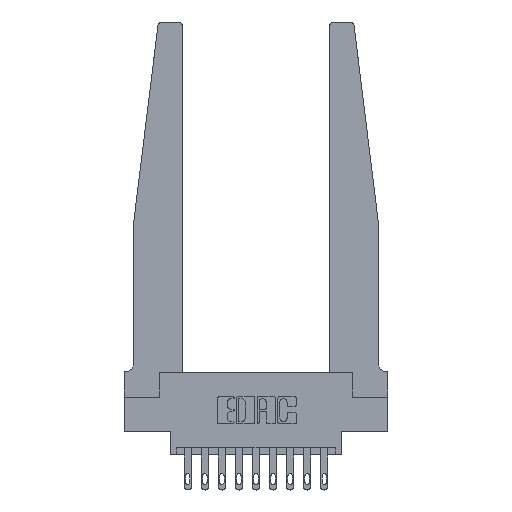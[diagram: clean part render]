
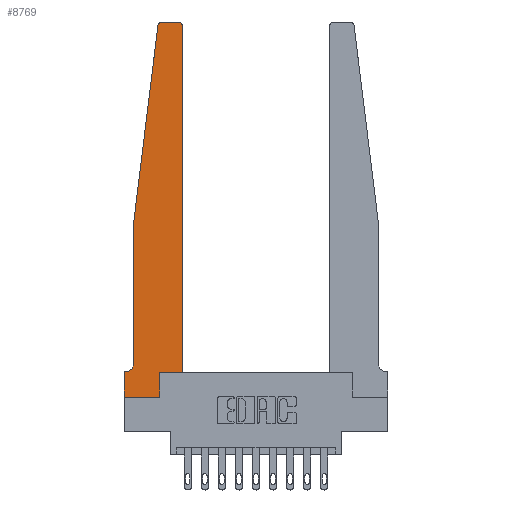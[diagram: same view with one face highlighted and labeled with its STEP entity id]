
A CAD part, top view. The second image highlights one B-rep face of the part: STEP entity #8769.
In plain terms, the highlighted planar face has unit normal (0, 0, 1).
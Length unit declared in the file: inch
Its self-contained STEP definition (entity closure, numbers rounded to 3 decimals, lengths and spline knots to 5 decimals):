
#278 = CARTESIAN_POINT ( 'NONE',  ( 0., 0.1875, 0.37 ) ) ;
#297 = CARTESIAN_POINT ( 'NONE',  ( 0.24675, 2.72367, 0.37 ) ) ;
#384 = DIRECTION ( 'NONE',  ( 0., 1., 0. ) ) ;
#623 = VERTEX_POINT ( 'NONE', #12539 ) ;
#627 = CARTESIAN_POINT ( 'NONE',  ( 0.425, 2.72, 0.37 ) ) ;
#632 = EDGE_CURVE ( 'NONE', #8275, #15040, #13407, .T. ) ;
#666 = VECTOR ( 'NONE', #12272, 39.37008 ) ;
#697 = CARTESIAN_POINT ( 'NONE',  ( 0.2605, 0.18, 0.37 ) ) ;
#800 = VERTEX_POINT ( 'NONE', #627 ) ;
#1110 = CIRCLE ( 'NONE', #4379, 0.05 ) ;
#1800 = DIRECTION ( 'NONE',  ( 0., 0., 1. ) ) ;
#1875 = CARTESIAN_POINT ( 'NONE',  ( 0.015, 0.1875, 0.37 ) ) ;
#2481 = CIRCLE ( 'NONE', #14041, 0.03 ) ;
#2810 = CARTESIAN_POINT ( 'NONE',  ( 0.395, 2.75, 0.37 ) ) ;
#2941 = ORIENTED_EDGE ( 'NONE', *, *, #6057, .T. ) ;
#2956 = DIRECTION ( 'NONE',  ( 1., 0., 0. ) ) ;
#3009 = CARTESIAN_POINT ( 'NONE',  ( 0.395, 2.72, 0.37 ) ) ;
#3151 = VECTOR ( 'NONE', #12362, 39.37008 ) ;
#3582 = CARTESIAN_POINT ( 'NONE',  ( 0.2605, 0.18, 0.37 ) ) ;
#3912 = AXIS2_PLACEMENT_3D ( 'NONE', #4189, #11306, #2956 ) ;
#4028 = ORIENTED_EDGE ( 'NONE', *, *, #6815, .T. ) ;
#4189 = CARTESIAN_POINT ( 'NONE',  ( 0., 0.1875, 0.37 ) ) ;
#4379 = AXIS2_PLACEMENT_3D ( 'NONE', #13967, #10591, #9338 ) ;
#4678 = LINE ( 'NONE', #3582, #14267 ) ;
#4982 = ORIENTED_EDGE ( 'NONE', *, *, #15145, .T. ) ;
#5058 = EDGE_CURVE ( 'NONE', #623, #11963, #1110, .T. ) ;
#5105 = LINE ( 'NONE', #10248, #3151 ) ;
#5292 = VERTEX_POINT ( 'NONE', #6308 ) ;
#5338 = CARTESIAN_POINT ( 'NONE',  ( 0.2605, 0., 0.37 ) ) ;
#5993 = DIRECTION ( 'NONE',  ( 1., 0., 0. ) ) ;
#6057 = EDGE_CURVE ( 'NONE', #9162, #15502, #8479, .T. ) ;
#6308 = CARTESIAN_POINT ( 'NONE',  ( 0., 0., 0.37 ) ) ;
#6447 = CARTESIAN_POINT ( 'NONE',  ( 0.27653, 2.72, 0.37 ) ) ;
#6736 = CARTESIAN_POINT ( 'NONE',  ( 0.065, 1.25, 0.37 ) ) ;
#6815 = EDGE_CURVE ( 'NONE', #5292, #9158, #13242, .T. ) ;
#7199 = AXIS2_PLACEMENT_3D ( 'NONE', #6447, #1800, #13536 ) ;
#7262 = VERTEX_POINT ( 'NONE', #9844 ) ;
#7490 = CARTESIAN_POINT ( 'NONE',  ( 0.425, 0.18, 0.37 ) ) ;
#7545 = VECTOR ( 'NONE', #9275, 39.37008 ) ;
#7759 = CARTESIAN_POINT ( 'NONE',  ( 0.065, 1.25, 0.37 ) ) ;
#7775 = CARTESIAN_POINT ( 'NONE',  ( 0.425, 0.18, 0.37 ) ) ;
#7809 = DIRECTION ( 'NONE',  ( 1., 0., 0. ) ) ;
#7975 = LINE ( 'NONE', #15061, #11849 ) ;
#7992 = LINE ( 'NONE', #14060, #7545 ) ;
#8072 = EDGE_CURVE ( 'NONE', #13817, #5292, #5105, .T. ) ;
#8135 = ORIENTED_EDGE ( 'NONE', *, *, #14205, .T. ) ;
#8151 = EDGE_CURVE ( 'NONE', #15040, #800, #11354, .T. ) ;
#8275 = VERTEX_POINT ( 'NONE', #697 ) ;
#8479 = LINE ( 'NONE', #7759, #14659 ) ;
#8769 = ADVANCED_FACE ( 'NONE', ( #10051 ), #9096, .T. ) ;
#8773 = CARTESIAN_POINT ( 'NONE',  ( 0.425, 0.18, 0.37 ) ) ;
#8933 = ORIENTED_EDGE ( 'NONE', *, *, #8072, .T. ) ;
#8971 = LINE ( 'NONE', #12194, #666 ) ;
#9096 = PLANE ( 'NONE',  #3912 ) ;
#9158 = VERTEX_POINT ( 'NONE', #5338 ) ;
#9162 = VERTEX_POINT ( 'NONE', #297 ) ;
#9275 = DIRECTION ( 'NONE',  ( -1., 0., 0. ) ) ;
#9338 = DIRECTION ( 'NONE',  ( -1., 0., 0. ) ) ;
#9795 = EDGE_LOOP ( 'NONE', ( #14945, #12251, #2941, #10811, #12853, #12075, #8933, #4028, #4982, #14151, #12246, #8135 ) ) ;
#9844 = CARTESIAN_POINT ( 'NONE',  ( 0.27653, 2.75, 0.37 ) ) ;
#9904 = VECTOR ( 'NONE', #5993, 39.37008 ) ;
#9949 = VECTOR ( 'NONE', #384, 39.37008 ) ;
#10051 = FACE_OUTER_BOUND ( 'NONE', #9795, .T. ) ;
#10126 = DIRECTION ( 'NONE',  ( -0.122, -0.992, 0. ) ) ;
#10190 = DIRECTION ( 'NONE',  ( 0., -1., 0. ) ) ;
#10248 = CARTESIAN_POINT ( 'NONE',  ( 0., 0., 0.37 ) ) ;
#10591 = DIRECTION ( 'NONE',  ( 0., 0., -1. ) ) ;
#10720 = CARTESIAN_POINT ( 'NONE',  ( 0., 0., 0.37 ) ) ;
#10738 = EDGE_CURVE ( 'NONE', #7262, #9162, #14754, .T. ) ;
#10811 = ORIENTED_EDGE ( 'NONE', *, *, #11702, .T. ) ;
#11174 = VERTEX_POINT ( 'NONE', #2810 ) ;
#11306 = DIRECTION ( 'NONE',  ( 0., 0., 1. ) ) ;
#11354 = LINE ( 'NONE', #8773, #9949 ) ;
#11370 = EDGE_CURVE ( 'NONE', #11174, #7262, #7992, .T. ) ;
#11702 = EDGE_CURVE ( 'NONE', #15502, #623, #7975, .T. ) ;
#11849 = VECTOR ( 'NONE', #10190, 39.37008 ) ;
#11935 = DIRECTION ( 'NONE',  ( 0., 1., 0. ) ) ;
#11963 = VERTEX_POINT ( 'NONE', #1875 ) ;
#12075 = ORIENTED_EDGE ( 'NONE', *, *, #14900, .T. ) ;
#12194 = CARTESIAN_POINT ( 'NONE',  ( 0.065, 0.1875, 0.37 ) ) ;
#12246 = ORIENTED_EDGE ( 'NONE', *, *, #8151, .T. ) ;
#12251 = ORIENTED_EDGE ( 'NONE', *, *, #10738, .T. ) ;
#12272 = DIRECTION ( 'NONE',  ( -1., 0., 0. ) ) ;
#12289 = VECTOR ( 'NONE', #14892, 39.37008 ) ;
#12362 = DIRECTION ( 'NONE',  ( 0., -1., 0. ) ) ;
#12539 = CARTESIAN_POINT ( 'NONE',  ( 0.065, 0.2375, 0.37 ) ) ;
#12540 = DIRECTION ( 'NONE',  ( 0., 0., 1. ) ) ;
#12853 = ORIENTED_EDGE ( 'NONE', *, *, #5058, .T. ) ;
#13242 = LINE ( 'NONE', #10720, #9904 ) ;
#13407 = LINE ( 'NONE', #7490, #12289 ) ;
#13536 = DIRECTION ( 'NONE',  ( 1., 0., 0. ) ) ;
#13817 = VERTEX_POINT ( 'NONE', #278 ) ;
#13967 = CARTESIAN_POINT ( 'NONE',  ( 0.015, 0.2375, 0.37 ) ) ;
#14041 = AXIS2_PLACEMENT_3D ( 'NONE', #3009, #12540, #7809 ) ;
#14060 = CARTESIAN_POINT ( 'NONE',  ( 0.25, 2.75, 0.37 ) ) ;
#14151 = ORIENTED_EDGE ( 'NONE', *, *, #632, .T. ) ;
#14205 = EDGE_CURVE ( 'NONE', #800, #11174, #2481, .T. ) ;
#14267 = VECTOR ( 'NONE', #11935, 39.37008 ) ;
#14659 = VECTOR ( 'NONE', #10126, 39.37008 ) ;
#14754 = CIRCLE ( 'NONE', #7199, 0.03 ) ;
#14892 = DIRECTION ( 'NONE',  ( 1., 0., 0. ) ) ;
#14900 = EDGE_CURVE ( 'NONE', #11963, #13817, #8971, .T. ) ;
#14945 = ORIENTED_EDGE ( 'NONE', *, *, #11370, .T. ) ;
#15040 = VERTEX_POINT ( 'NONE', #7775 ) ;
#15061 = CARTESIAN_POINT ( 'NONE',  ( 0.065, 1.25, 0.37 ) ) ;
#15145 = EDGE_CURVE ( 'NONE', #9158, #8275, #4678, .T. ) ;
#15502 = VERTEX_POINT ( 'NONE', #6736 ) ;
